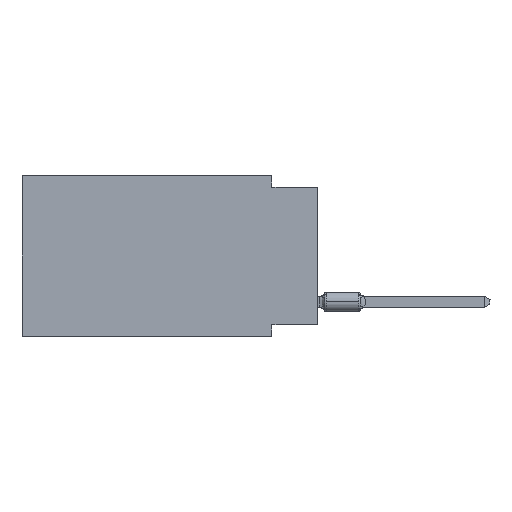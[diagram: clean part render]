
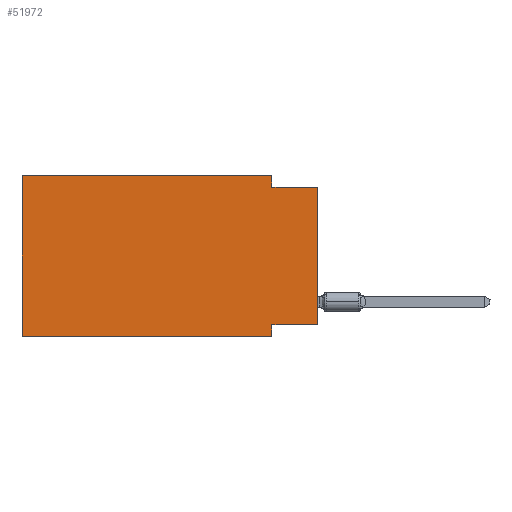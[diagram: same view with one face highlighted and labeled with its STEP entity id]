
A CAD part, left-side view. The second image highlights one B-rep face of the part: STEP entity #51972.
In plain terms, the highlighted planar face has unit normal (-1, 0, 0).
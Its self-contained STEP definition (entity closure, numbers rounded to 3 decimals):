
#2337 = DIRECTION ( 'NONE',  ( 0., 0., -1. ) ) ;
#3956 = CARTESIAN_POINT ( 'NONE',  ( 0., 2.54, -0.635 ) ) ;
#4853 = EDGE_CURVE ( 'NONE', #28318, #12487, #61957, .T. ) ;
#5323 = CARTESIAN_POINT ( 'NONE',  ( 0., 16.383, -8.89 ) ) ;
#6104 = FACE_OUTER_BOUND ( 'NONE', #35535, .T. ) ;
#6238 = LINE ( 'NONE', #6727, #75600 ) ;
#6727 = CARTESIAN_POINT ( 'NONE',  ( 0., 0., 0. ) ) ;
#7092 = CARTESIAN_POINT ( 'NONE',  ( 0., 0., -8.255 ) ) ;
#7809 = ORIENTED_EDGE ( 'NONE', *, *, #57288, .F. ) ;
#8405 = DIRECTION ( 'NONE',  ( 0., -1., 0. ) ) ;
#12404 = CARTESIAN_POINT ( 'NONE',  ( 0., 2.54, 0. ) ) ;
#12487 = VERTEX_POINT ( 'NONE', #42975 ) ;
#13254 = DIRECTION ( 'NONE',  ( 0., 0., -1. ) ) ;
#15530 = CARTESIAN_POINT ( 'NONE',  ( 0., 16.383, 0. ) ) ;
#15584 = ORIENTED_EDGE ( 'NONE', *, *, #40240, .T. ) ;
#17407 = VERTEX_POINT ( 'NONE', #88243 ) ;
#19354 = VECTOR ( 'NONE', #91282, 1000. ) ;
#20756 = DIRECTION ( 'NONE',  ( 0., 0., -1. ) ) ;
#21069 = CARTESIAN_POINT ( 'NONE',  ( 0., 2.54, -8.89 ) ) ;
#24700 = VECTOR ( 'NONE', #42505, 1000. ) ;
#28318 = VERTEX_POINT ( 'NONE', #5323 ) ;
#28994 = CARTESIAN_POINT ( 'NONE',  ( 0., 0., -8.255 ) ) ;
#30523 = LINE ( 'NONE', #7092, #43825 ) ;
#30612 = ORIENTED_EDGE ( 'NONE', *, *, #58798, .F. ) ;
#35535 = EDGE_LOOP ( 'NONE', ( #15584, #59564, #30612, #93517, #87951, #73309, #7809, #71614 ) ) ;
#36070 = DIRECTION ( 'NONE',  ( 0., -1., 0. ) ) ;
#36543 = DIRECTION ( 'NONE',  ( 0., 0., 1. ) ) ;
#37238 = CARTESIAN_POINT ( 'NONE',  ( 0., 16.383, -8.89 ) ) ;
#40240 = EDGE_CURVE ( 'NONE', #43628, #17407, #6238, .T. ) ;
#41428 = EDGE_CURVE ( 'NONE', #12487, #83022, #52189, .T. ) ;
#42505 = DIRECTION ( 'NONE',  ( 0., -1., 0. ) ) ;
#42975 = CARTESIAN_POINT ( 'NONE',  ( 0., 16.383, 0. ) ) ;
#43243 = DIRECTION ( 'NONE',  ( 1., 0., 0. ) ) ;
#43305 = CARTESIAN_POINT ( 'NONE',  ( 0., 2.54, -8.89 ) ) ;
#43628 = VERTEX_POINT ( 'NONE', #28994 ) ;
#43825 = VECTOR ( 'NONE', #44710, 1000. ) ;
#44710 = DIRECTION ( 'NONE',  ( 0., 1., 0. ) ) ;
#48208 = EDGE_CURVE ( 'NONE', #43628, #77778, #30523, .T. ) ;
#51972 = ADVANCED_FACE ( 'NONE', ( #6104 ), #87211, .F. ) ;
#52189 = LINE ( 'NONE', #15530, #78715 ) ;
#54778 = VERTEX_POINT ( 'NONE', #3956 ) ;
#55141 = LINE ( 'NONE', #37238, #66306 ) ;
#56807 = VECTOR ( 'NONE', #2337, 1000. ) ;
#56872 = LINE ( 'NONE', #12404, #56807 ) ;
#56899 = VERTEX_POINT ( 'NONE', #43305 ) ;
#57288 = EDGE_CURVE ( 'NONE', #77778, #56899, #96302, .T. ) ;
#58798 = EDGE_CURVE ( 'NONE', #83022, #54778, #56872, .T. ) ;
#59564 = ORIENTED_EDGE ( 'NONE', *, *, #82424, .F. ) ;
#59697 = EDGE_CURVE ( 'NONE', #28318, #56899, #55141, .T. ) ;
#61957 = LINE ( 'NONE', #91761, #19354 ) ;
#65951 = CARTESIAN_POINT ( 'NONE',  ( 0., 0., -0.635 ) ) ;
#66306 = VECTOR ( 'NONE', #8405, 1000. ) ;
#67716 = CARTESIAN_POINT ( 'NONE',  ( 0., 2.54, -8.255 ) ) ;
#71614 = ORIENTED_EDGE ( 'NONE', *, *, #48208, .F. ) ;
#73309 = ORIENTED_EDGE ( 'NONE', *, *, #59697, .T. ) ;
#73529 = CARTESIAN_POINT ( 'NONE',  ( 0., 16.383, 0. ) ) ;
#75600 = VECTOR ( 'NONE', #36543, 1000. ) ;
#76928 = VECTOR ( 'NONE', #13254, 1000. ) ;
#77778 = VERTEX_POINT ( 'NONE', #67716 ) ;
#78715 = VECTOR ( 'NONE', #36070, 1000. ) ;
#80624 = LINE ( 'NONE', #65951, #24700 ) ;
#82424 = EDGE_CURVE ( 'NONE', #54778, #17407, #80624, .T. ) ;
#83022 = VERTEX_POINT ( 'NONE', #89758 ) ;
#87211 = PLANE ( 'NONE',  #91139 ) ;
#87951 = ORIENTED_EDGE ( 'NONE', *, *, #4853, .F. ) ;
#88243 = CARTESIAN_POINT ( 'NONE',  ( 0., 0., -0.635 ) ) ;
#89758 = CARTESIAN_POINT ( 'NONE',  ( 0., 2.54, 0. ) ) ;
#91139 = AXIS2_PLACEMENT_3D ( 'NONE', #73529, #43243, #20756 ) ;
#91282 = DIRECTION ( 'NONE',  ( 0., 0., 1. ) ) ;
#91761 = CARTESIAN_POINT ( 'NONE',  ( 0., 16.383, 0. ) ) ;
#93517 = ORIENTED_EDGE ( 'NONE', *, *, #41428, .F. ) ;
#96302 = LINE ( 'NONE', #21069, #76928 ) ;
